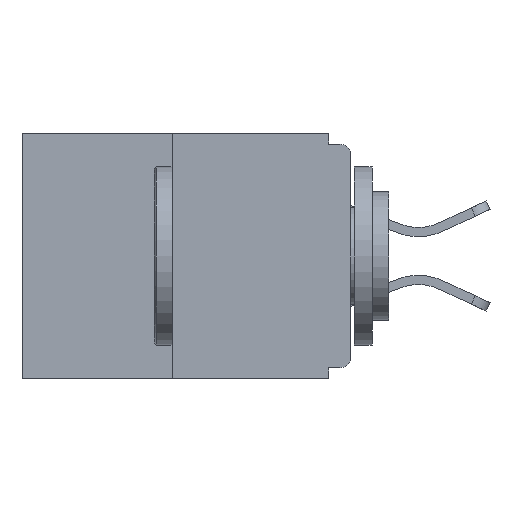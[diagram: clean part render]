
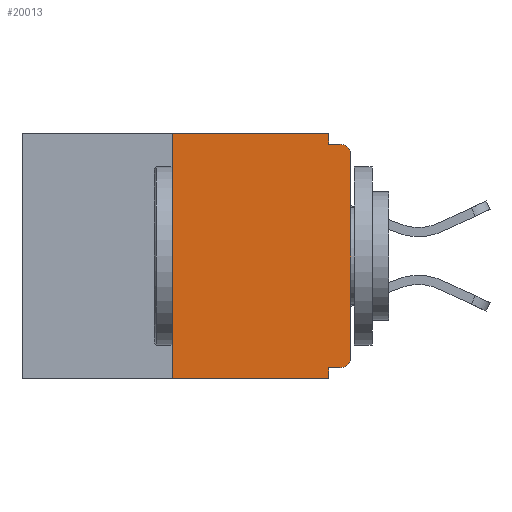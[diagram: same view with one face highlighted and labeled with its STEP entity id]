
A CAD part, left-side view. The second image highlights one B-rep face of the part: STEP entity #20013.
In plain terms, the highlighted planar face has unit normal (-1, 0, 0).
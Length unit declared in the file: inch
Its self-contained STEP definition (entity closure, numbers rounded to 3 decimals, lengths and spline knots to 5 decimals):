
#252 = CARTESIAN_POINT ( 'NONE',  ( 0., 0., -0.313 ) ) ;
#461 = VECTOR ( 'NONE', #8785, 39.37008 ) ;
#723 = CARTESIAN_POINT ( 'NONE',  ( 0., 0.46, -0.343 ) ) ;
#1113 = DIRECTION ( 'NONE',  ( 0., 0., -1. ) ) ;
#1318 = LINE ( 'NONE', #10912, #16784 ) ;
#1806 = LINE ( 'NONE', #15331, #7713 ) ;
#2298 = DIRECTION ( 'NONE',  ( 0., 0., -1. ) ) ;
#2337 = VERTEX_POINT ( 'NONE', #8062 ) ;
#2396 = CARTESIAN_POINT ( 'NONE',  ( 0., 0.031, 0. ) ) ;
#2468 = DIRECTION ( 'NONE',  ( 0., 0., -1. ) ) ;
#3519 = DIRECTION ( 'NONE',  ( 0., 0., -1. ) ) ;
#3606 = ORIENTED_EDGE ( 'NONE', *, *, #19407, .F. ) ;
#3718 = EDGE_CURVE ( 'NONE', #10326, #5775, #1806, .T. ) ;
#4237 = EDGE_CURVE ( 'NONE', #10326, #25413, #20713, .T. ) ;
#4590 = VECTOR ( 'NONE', #6276, 39.37008 ) ;
#4870 = ORIENTED_EDGE ( 'NONE', *, *, #4237, .T. ) ;
#5158 = CARTESIAN_POINT ( 'NONE',  ( 0., 0.25, 0. ) ) ;
#5172 = ORIENTED_EDGE ( 'NONE', *, *, #3718, .F. ) ;
#5332 = CARTESIAN_POINT ( 'NONE',  ( 0., 0., -0.015 ) ) ;
#5453 = AXIS2_PLACEMENT_3D ( 'NONE', #25053, #19121, #3519 ) ;
#5460 = CARTESIAN_POINT ( 'NONE',  ( 0., 0.031, -0.328 ) ) ;
#5775 = VERTEX_POINT ( 'NONE', #5460 ) ;
#5791 = ORIENTED_EDGE ( 'NONE', *, *, #11051, .F. ) ;
#6276 = DIRECTION ( 'NONE',  ( 0., 0., -1. ) ) ;
#6559 = ORIENTED_EDGE ( 'NONE', *, *, #23500, .F. ) ;
#6883 = VERTEX_POINT ( 'NONE', #2396 ) ;
#7713 = VECTOR ( 'NONE', #19500, 39.37008 ) ;
#7722 = VERTEX_POINT ( 'NONE', #11604 ) ;
#7999 = LINE ( 'NONE', #12216, #4590 ) ;
#8032 = DIRECTION ( 'NONE',  ( 1., 0., 0. ) ) ;
#8062 = CARTESIAN_POINT ( 'NONE',  ( 0., 0.031, -0.015 ) ) ;
#8194 = EDGE_LOOP ( 'NONE', ( #25620, #23907, #14876, #3606, #5172, #4870, #19503, #25070, #6559, #5791 ) ) ;
#8626 = CARTESIAN_POINT ( 'NONE',  ( 0., 0.25, 0. ) ) ;
#8785 = DIRECTION ( 'NONE',  ( 0., 0., 1. ) ) ;
#8960 = EDGE_CURVE ( 'NONE', #25413, #15526, #10119, .T. ) ;
#9837 = CARTESIAN_POINT ( 'NONE',  ( 0., 0., 0. ) ) ;
#9938 = EDGE_CURVE ( 'NONE', #18490, #18303, #16554, .T. ) ;
#10119 = LINE ( 'NONE', #9837, #20370 ) ;
#10326 = VERTEX_POINT ( 'NONE', #11623 ) ;
#10581 = VECTOR ( 'NONE', #14319, 39.37008 ) ;
#10912 = CARTESIAN_POINT ( 'NONE',  ( 0., 0.031, 0. ) ) ;
#11051 = EDGE_CURVE ( 'NONE', #6883, #2337, #1318, .T. ) ;
#11427 = CARTESIAN_POINT ( 'NONE',  ( 0., 0., -0.03 ) ) ;
#11566 = CARTESIAN_POINT ( 'NONE',  ( 0., 0.25, -0.343 ) ) ;
#11604 = CARTESIAN_POINT ( 'NONE',  ( 0., 0.031, -0.343 ) ) ;
#11623 = CARTESIAN_POINT ( 'NONE',  ( 0., 0.015, -0.328 ) ) ;
#11650 = DIRECTION ( 'NONE',  ( 0., 0., 1. ) ) ;
#12216 = CARTESIAN_POINT ( 'NONE',  ( 0., 0.031, -0.343 ) ) ;
#12397 = CARTESIAN_POINT ( 'NONE',  ( 0., 0.015, -0.015 ) ) ;
#12902 = CIRCLE ( 'NONE', #5453, 0.015 ) ;
#13191 = AXIS2_PLACEMENT_3D ( 'NONE', #15888, #8032, #2298 ) ;
#14319 = DIRECTION ( 'NONE',  ( 0., -1., 0. ) ) ;
#14876 = ORIENTED_EDGE ( 'NONE', *, *, #24188, .T. ) ;
#15331 = CARTESIAN_POINT ( 'NONE',  ( 0., 0., -0.328 ) ) ;
#15500 = CARTESIAN_POINT ( 'NONE',  ( 0., 0.46, 0. ) ) ;
#15526 = VERTEX_POINT ( 'NONE', #11427 ) ;
#15888 = CARTESIAN_POINT ( 'NONE',  ( 0., 0.46, 0. ) ) ;
#16554 = LINE ( 'NONE', #5158, #461 ) ;
#16579 = CARTESIAN_POINT ( 'NONE',  ( 0., 0.015, -0.313 ) ) ;
#16784 = VECTOR ( 'NONE', #1113, 39.37008 ) ;
#16934 = FACE_OUTER_BOUND ( 'NONE', #8194, .T. ) ;
#17999 = LINE ( 'NONE', #723, #10581 ) ;
#18303 = VERTEX_POINT ( 'NONE', #8626 ) ;
#18490 = VERTEX_POINT ( 'NONE', #11566 ) ;
#18587 = DIRECTION ( 'NONE',  ( -1., 0., 0. ) ) ;
#19121 = DIRECTION ( 'NONE',  ( -1., 0., 0. ) ) ;
#19407 = EDGE_CURVE ( 'NONE', #5775, #7722, #7999, .T. ) ;
#19500 = DIRECTION ( 'NONE',  ( 0., 1., 0. ) ) ;
#19503 = ORIENTED_EDGE ( 'NONE', *, *, #8960, .T. ) ;
#19586 = DIRECTION ( 'NONE',  ( 0., -1., 0. ) ) ;
#20013 = ADVANCED_FACE ( 'NONE', ( #16934 ), #23924, .F. ) ;
#20193 = VECTOR ( 'NONE', #19586, 39.37008 ) ;
#20295 = AXIS2_PLACEMENT_3D ( 'NONE', #16579, #18587, #2468 ) ;
#20370 = VECTOR ( 'NONE', #11650, 39.37008 ) ;
#20713 = CIRCLE ( 'NONE', #20295, 0.015 ) ;
#20918 = EDGE_CURVE ( 'NONE', #15526, #21970, #12902, .T. ) ;
#21970 = VERTEX_POINT ( 'NONE', #12397 ) ;
#22952 = DIRECTION ( 'NONE',  ( 0., -1., 0. ) ) ;
#23500 = EDGE_CURVE ( 'NONE', #2337, #21970, #24537, .T. ) ;
#23907 = ORIENTED_EDGE ( 'NONE', *, *, #9938, .F. ) ;
#23924 = PLANE ( 'NONE',  #13191 ) ;
#24188 = EDGE_CURVE ( 'NONE', #18490, #7722, #17999, .T. ) ;
#24537 = LINE ( 'NONE', #5332, #25460 ) ;
#24585 = EDGE_CURVE ( 'NONE', #18303, #6883, #25403, .T. ) ;
#25053 = CARTESIAN_POINT ( 'NONE',  ( 0., 0.015, -0.03 ) ) ;
#25070 = ORIENTED_EDGE ( 'NONE', *, *, #20918, .T. ) ;
#25403 = LINE ( 'NONE', #15500, #20193 ) ;
#25413 = VERTEX_POINT ( 'NONE', #252 ) ;
#25460 = VECTOR ( 'NONE', #22952, 39.37008 ) ;
#25620 = ORIENTED_EDGE ( 'NONE', *, *, #24585, .F. ) ;
